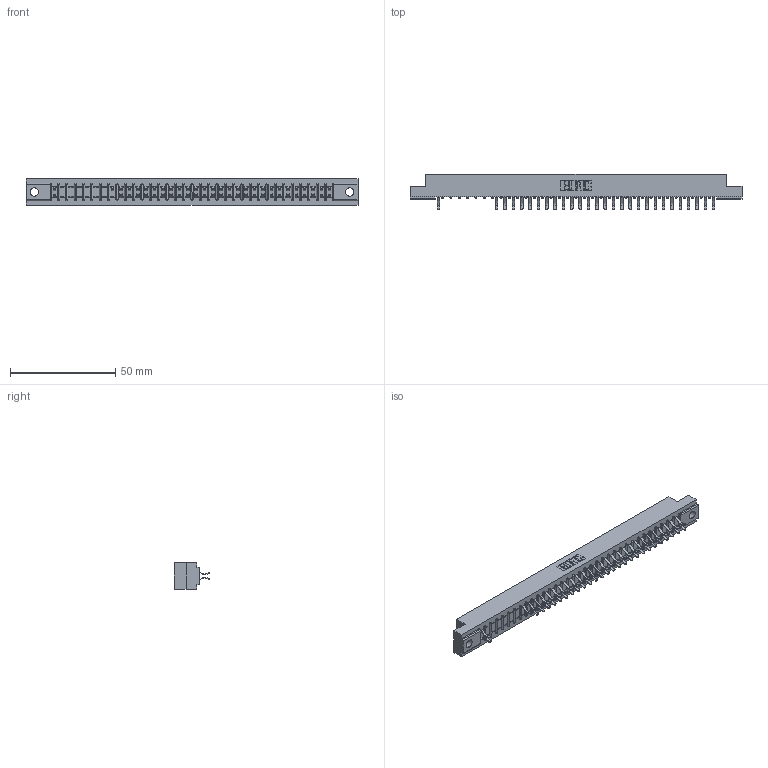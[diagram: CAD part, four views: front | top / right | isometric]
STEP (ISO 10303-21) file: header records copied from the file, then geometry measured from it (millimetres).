
FILE_DESCRIPTION (( 'STEP AP203' ), '1' );
FILE_NAME ('307-068-556-204.STEP', '2018-08-06T12:15:52', ( '' ), ( '' ), 'SwSTEP 2.0', 'SolidWorks 2016', '' );
FILE_SCHEMA (( 'CONFIG_CONTROL_DESIGN' ));
Length unit declared in the file: inch
Products named in the file (3): 307 Part_.156 Dia Mounting Holes; 307-290-001_556; 307-068-556-204
Assembly tree (56 placements, depth 2):
  307-068-556-204
    307 Part_.156 Dia Mounting Holes
    307-290-001_556  x55
Bounding box: 157.73 x 16.97 x 12.7 mm (x, y, z)
Volume: 16432.2 mm3; surface area: 18527.6 mm2
Topology: 56 solids, 56 shells, 3047 faces, 8585 edges, 5554 vertices
Faces by surface type: plane 1977, cylinder 1000, sphere 70
Entity records: 31328 total; most frequent: CARTESIAN_POINT 5187, ORIENTED_EDGE 5150, DIRECTION 5063, EDGE_CURVE 2575, LINE 1979, VECTOR 1979, VERTEX_POINT 1666, AXIS2_PLACEMENT_3D 1542
